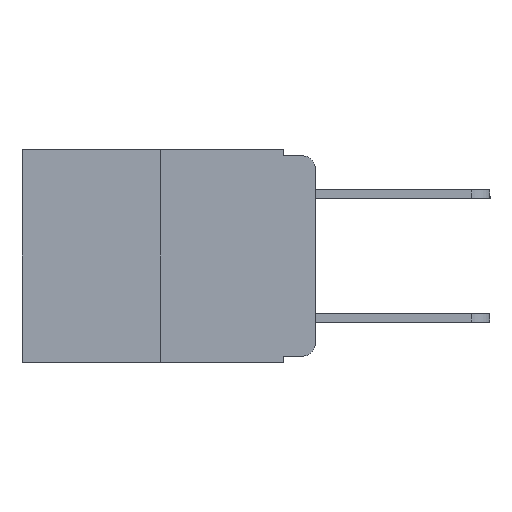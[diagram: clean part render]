
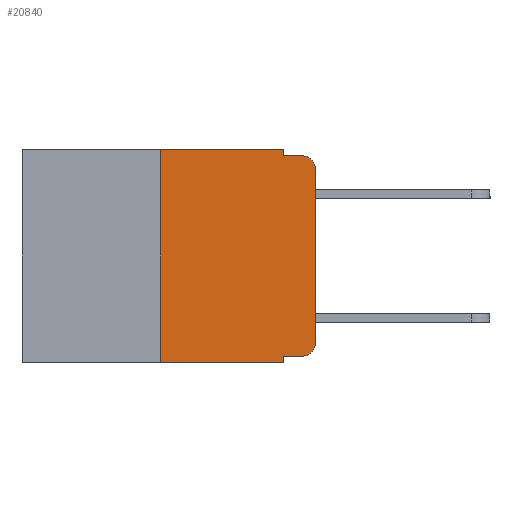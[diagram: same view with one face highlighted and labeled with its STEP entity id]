
A CAD part, left-side view. The second image highlights one B-rep face of the part: STEP entity #20840.
In plain terms, the highlighted planar face has unit normal (-1, 0, 0).
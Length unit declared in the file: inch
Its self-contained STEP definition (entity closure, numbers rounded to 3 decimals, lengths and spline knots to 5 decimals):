
#8 = DIRECTION ( 'NONE',  ( -1., 0., 0. ) ) ;
#473 = DIRECTION ( 'NONE',  ( 0., -1., 0. ) ) ;
#640 = CARTESIAN_POINT ( 'NONE',  ( 0., 0.051, -0.333 ) ) ;
#1591 = VERTEX_POINT ( 'NONE', #4341 ) ;
#1644 = DIRECTION ( 'NONE',  ( 0., -1., 0. ) ) ;
#1773 = ORIENTED_EDGE ( 'NONE', *, *, #19281, .T. ) ;
#1867 = CARTESIAN_POINT ( 'NONE',  ( 0., 0.02, -0.333 ) ) ;
#2100 = VECTOR ( 'NONE', #20627, 39.37008 ) ;
#2308 = VERTEX_POINT ( 'NONE', #13815 ) ;
#2459 = CARTESIAN_POINT ( 'NONE',  ( 0., 0., -0.03 ) ) ;
#3115 = LINE ( 'NONE', #13284, #17816 ) ;
#3118 = LINE ( 'NONE', #5556, #22680 ) ;
#3279 = DIRECTION ( 'NONE',  ( 1., 0., 0. ) ) ;
#3337 = CARTESIAN_POINT ( 'NONE',  ( 0., 0., -0.313 ) ) ;
#3475 = EDGE_CURVE ( 'NONE', #5729, #11928, #21691, .T. ) ;
#4135 = CARTESIAN_POINT ( 'NONE',  ( 0., 0.051, 0. ) ) ;
#4341 = CARTESIAN_POINT ( 'NONE',  ( 0., 0.02, -0.01 ) ) ;
#4637 = VERTEX_POINT ( 'NONE', #3337 ) ;
#4851 = LINE ( 'NONE', #12695, #23732 ) ;
#5224 = ORIENTED_EDGE ( 'NONE', *, *, #22503, .T. ) ;
#5556 = CARTESIAN_POINT ( 'NONE',  ( 0., 0.473, -0.343 ) ) ;
#5729 = VERTEX_POINT ( 'NONE', #16869 ) ;
#6515 = AXIS2_PLACEMENT_3D ( 'NONE', #10934, #3279, #16718 ) ;
#6907 = DIRECTION ( 'NONE',  ( -1., 0., 0. ) ) ;
#6931 = DIRECTION ( 'NONE',  ( 0., 0., 1. ) ) ;
#7300 = EDGE_CURVE ( 'NONE', #11928, #1591, #21779, .T. ) ;
#7819 = CARTESIAN_POINT ( 'NONE',  ( 0., 0.051, -0.343 ) ) ;
#7900 = ORIENTED_EDGE ( 'NONE', *, *, #20205, .F. ) ;
#8319 = VERTEX_POINT ( 'NONE', #2459 ) ;
#8597 = EDGE_CURVE ( 'NONE', #10189, #2308, #4851, .T. ) ;
#9245 = CARTESIAN_POINT ( 'NONE',  ( 0., 0.051, -0.01 ) ) ;
#9472 = CARTESIAN_POINT ( 'NONE',  ( 0., 0., 0. ) ) ;
#9651 = VERTEX_POINT ( 'NONE', #640 ) ;
#10189 = VERTEX_POINT ( 'NONE', #11651 ) ;
#10633 = CARTESIAN_POINT ( 'NONE',  ( 0., 0.051, -0.01 ) ) ;
#10934 = CARTESIAN_POINT ( 'NONE',  ( 0., 0.473, 0. ) ) ;
#11627 = DIRECTION ( 'NONE',  ( 0., 0., -1. ) ) ;
#11651 = CARTESIAN_POINT ( 'NONE',  ( 0., 0.25, -0.343 ) ) ;
#11830 = CARTESIAN_POINT ( 'NONE',  ( 0., 0.02, -0.313 ) ) ;
#11928 = VERTEX_POINT ( 'NONE', #10633 ) ;
#12695 = CARTESIAN_POINT ( 'NONE',  ( 0., 0.25, 0. ) ) ;
#13284 = CARTESIAN_POINT ( 'NONE',  ( 0., 0.473, 0. ) ) ;
#13584 = EDGE_CURVE ( 'NONE', #2308, #5729, #3115, .T. ) ;
#13709 = DIRECTION ( 'NONE',  ( 0., 0., -1. ) ) ;
#13815 = CARTESIAN_POINT ( 'NONE',  ( 0., 0.25, 0. ) ) ;
#14229 = EDGE_CURVE ( 'NONE', #4637, #8319, #14837, .T. ) ;
#14319 = LINE ( 'NONE', #23348, #23557 ) ;
#14552 = AXIS2_PLACEMENT_3D ( 'NONE', #18354, #6907, #20201 ) ;
#14837 = LINE ( 'NONE', #9472, #23478 ) ;
#14990 = EDGE_LOOP ( 'NONE', ( #15423, #1773, #17767, #22632, #15139, #21225, #17493, #7900, #23480, #5224 ) ) ;
#15139 = ORIENTED_EDGE ( 'NONE', *, *, #13584, .F. ) ;
#15228 = EDGE_CURVE ( 'NONE', #9651, #20449, #14319, .T. ) ;
#15423 = ORIENTED_EDGE ( 'NONE', *, *, #14229, .T. ) ;
#15945 = EDGE_CURVE ( 'NONE', #10189, #23583, #3118, .T. ) ;
#16718 = DIRECTION ( 'NONE',  ( 0., 0., -1. ) ) ;
#16869 = CARTESIAN_POINT ( 'NONE',  ( 0., 0.051, 0. ) ) ;
#17056 = LINE ( 'NONE', #23616, #24470 ) ;
#17388 = VECTOR ( 'NONE', #11627, 39.37008 ) ;
#17493 = ORIENTED_EDGE ( 'NONE', *, *, #15945, .T. ) ;
#17767 = ORIENTED_EDGE ( 'NONE', *, *, #7300, .F. ) ;
#17816 = VECTOR ( 'NONE', #24407, 39.37008 ) ;
#18113 = DIRECTION ( 'NONE',  ( 0., 0., -1. ) ) ;
#18185 = FACE_OUTER_BOUND ( 'NONE', #14990, .T. ) ;
#18229 = AXIS2_PLACEMENT_3D ( 'NONE', #11830, #8, #13709 ) ;
#18354 = CARTESIAN_POINT ( 'NONE',  ( 0., 0.02, -0.03 ) ) ;
#18518 = PLANE ( 'NONE',  #6515 ) ;
#19281 = EDGE_CURVE ( 'NONE', #8319, #1591, #20857, .T. ) ;
#20201 = DIRECTION ( 'NONE',  ( 0., 0., -1. ) ) ;
#20205 = EDGE_CURVE ( 'NONE', #9651, #23583, #17056, .T. ) ;
#20449 = VERTEX_POINT ( 'NONE', #1867 ) ;
#20627 = DIRECTION ( 'NONE',  ( 0., -1., 0. ) ) ;
#20840 = ADVANCED_FACE ( 'NONE', ( #18185 ), #18518, .F. ) ;
#20857 = CIRCLE ( 'NONE', #14552, 0.02 ) ;
#21225 = ORIENTED_EDGE ( 'NONE', *, *, #8597, .F. ) ;
#21691 = LINE ( 'NONE', #4135, #17388 ) ;
#21779 = LINE ( 'NONE', #9245, #2100 ) ;
#22109 = DIRECTION ( 'NONE',  ( 0., 0., 1. ) ) ;
#22503 = EDGE_CURVE ( 'NONE', #20449, #4637, #22943, .T. ) ;
#22632 = ORIENTED_EDGE ( 'NONE', *, *, #3475, .F. ) ;
#22680 = VECTOR ( 'NONE', #1644, 39.37008 ) ;
#22943 = CIRCLE ( 'NONE', #18229, 0.02 ) ;
#23348 = CARTESIAN_POINT ( 'NONE',  ( 0., 0.051, -0.333 ) ) ;
#23478 = VECTOR ( 'NONE', #6931, 39.37008 ) ;
#23480 = ORIENTED_EDGE ( 'NONE', *, *, #15228, .T. ) ;
#23557 = VECTOR ( 'NONE', #473, 39.37008 ) ;
#23583 = VERTEX_POINT ( 'NONE', #7819 ) ;
#23616 = CARTESIAN_POINT ( 'NONE',  ( 0., 0.051, 0. ) ) ;
#23732 = VECTOR ( 'NONE', #22109, 39.37008 ) ;
#24407 = DIRECTION ( 'NONE',  ( 0., -1., 0. ) ) ;
#24470 = VECTOR ( 'NONE', #18113, 39.37008 ) ;
